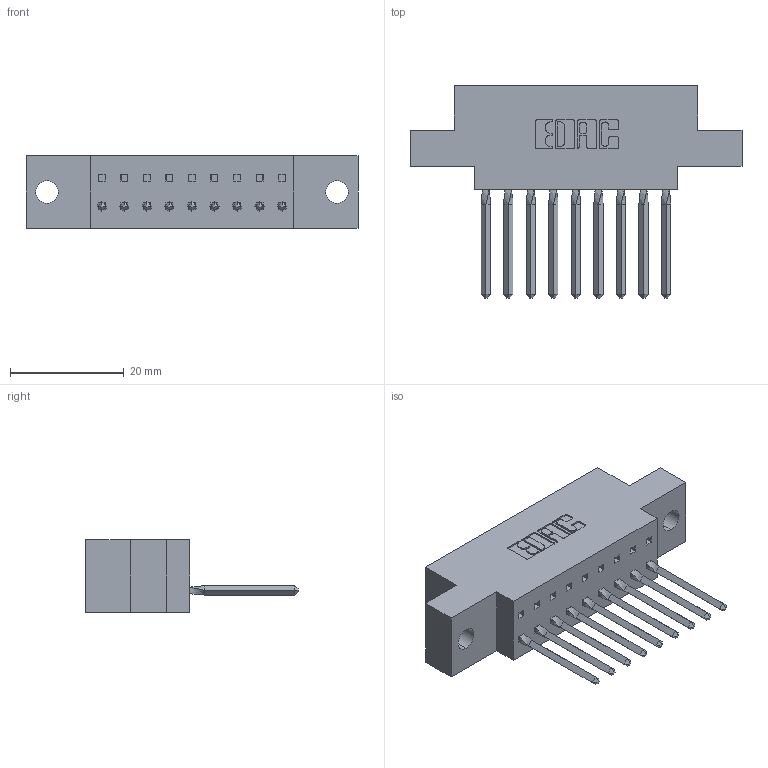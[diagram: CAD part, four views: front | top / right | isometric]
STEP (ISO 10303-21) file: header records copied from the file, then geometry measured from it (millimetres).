
FILE_DESCRIPTION (( 'STEP AP203' ), '1' );
FILE_NAME ('317-009-541-604.STEP', '2020-02-27T13:22:09', ( '' ), ( '' ), 'SwSTEP 2.0', 'SolidWorks 2016', '' );
FILE_SCHEMA (( 'CONFIG_CONTROL_DESIGN' ));
Length unit declared in the file: inch
Products named in the file (3): 317-290-002_541; 317-009-541-604; 317 Part_.156 Dia - TH
Assembly tree (10 placements, depth 2):
  317-009-541-604
    317 Part_.156 Dia - TH
    317-290-002_541  x9
Bounding box: 58.37 x 37.34 x 12.7 mm (x, y, z)
Volume: 8363 mm3; surface area: 10535.2 mm2
Topology: 10 solids, 10 shells, 1470 faces, 4181 edges, 2720 vertices
Faces by surface type: plane 1174, cylinder 260, bspline 36
Entity records: 18876 total; most frequent: CARTESIAN_POINT 3980, ORIENTED_EDGE 3242, DIRECTION 2639, EDGE_CURVE 1621, LINE 1257, VECTOR 1257, VERTEX_POINT 1072, AXIS2_PLACEMENT_3D 691
